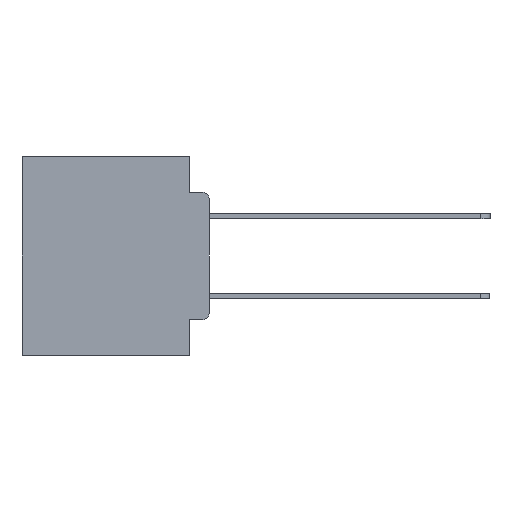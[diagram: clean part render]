
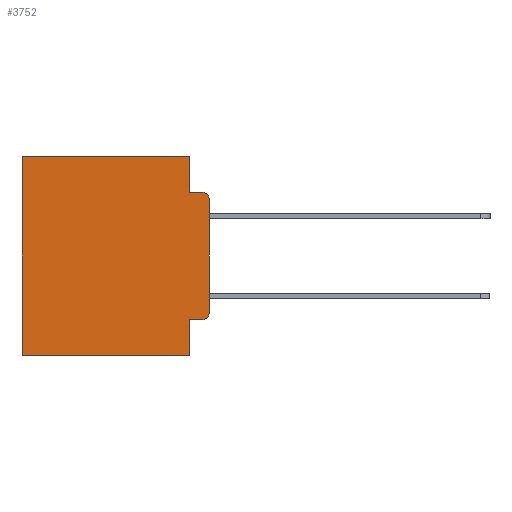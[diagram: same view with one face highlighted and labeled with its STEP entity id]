
A CAD part, left-side view. The second image highlights one B-rep face of the part: STEP entity #3752.
In plain terms, the highlighted planar face has unit normal (-1, 0, 0).
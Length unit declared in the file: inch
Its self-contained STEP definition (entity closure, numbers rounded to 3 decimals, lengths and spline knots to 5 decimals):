
#429 = CARTESIAN_POINT ( 'NONE',  ( 0.298, 0., -0.1085 ) ) ;
#691 = VECTOR ( 'NONE', #7239, 39.37008 ) ;
#1115 = ORIENTED_EDGE ( 'NONE', *, *, #2451, .T. ) ;
#2250 = CARTESIAN_POINT ( 'NONE',  ( 0.298, 0.473, 0. ) ) ;
#2272 = LINE ( 'NONE', #19275, #691 ) ;
#2451 = EDGE_CURVE ( 'NONE', #23999, #26126, #15797, .T. ) ;
#2770 = DIRECTION ( 'NONE',  ( -1., 0., 0. ) ) ;
#2798 = CARTESIAN_POINT ( 'NONE',  ( 0.298, 0., 0. ) ) ;
#3145 = ORIENTED_EDGE ( 'NONE', *, *, #28046, .T. ) ;
#3311 = DIRECTION ( 'NONE',  ( 0., 1., 0. ) ) ;
#3649 = EDGE_LOOP ( 'NONE', ( #17218, #3145, #24891, #10962, #20276, #14297, #28749, #30185, #22831, #1115 ) ) ;
#3752 = ADVANCED_FACE ( 'NONE', ( #28110 ), #26396, .F. ) ;
#4441 = AXIS2_PLACEMENT_3D ( 'NONE', #21143, #28683, #28322 ) ;
#5782 = EDGE_CURVE ( 'NONE', #24346, #23999, #2272, .T. ) ;
#5979 = DIRECTION ( 'NONE',  ( 0., 0., -1. ) ) ;
#6284 = CARTESIAN_POINT ( 'NONE',  ( 0.298, 0.051, -0.0885 ) ) ;
#6443 = DIRECTION ( 'NONE',  ( 0., 0., -1. ) ) ;
#6821 = CARTESIAN_POINT ( 'NONE',  ( 0.298, 0.051, -0.0885 ) ) ;
#7239 = DIRECTION ( 'NONE',  ( 0., -1., 0. ) ) ;
#7537 = LINE ( 'NONE', #23138, #25719 ) ;
#8365 = DIRECTION ( 'NONE',  ( -1., 0., 0. ) ) ;
#8428 = EDGE_CURVE ( 'NONE', #30101, #26126, #12114, .T. ) ;
#8796 = VERTEX_POINT ( 'NONE', #26924 ) ;
#9037 = EDGE_CURVE ( 'NONE', #24346, #30739, #7537, .T. ) ;
#9286 = DIRECTION ( 'NONE',  ( 0., -1., 0. ) ) ;
#10211 = DIRECTION ( 'NONE',  ( 0., 0., -1. ) ) ;
#10731 = EDGE_CURVE ( 'NONE', #30165, #25965, #17637, .T. ) ;
#10962 = ORIENTED_EDGE ( 'NONE', *, *, #18756, .F. ) ;
#11138 = DIRECTION ( 'NONE',  ( 0., 1., 0. ) ) ;
#12114 = LINE ( 'NONE', #2798, #23971 ) ;
#12420 = LINE ( 'NONE', #26131, #24270 ) ;
#13911 = EDGE_CURVE ( 'NONE', #25965, #8796, #14482, .T. ) ;
#14201 = VECTOR ( 'NONE', #9286, 39.37008 ) ;
#14297 = ORIENTED_EDGE ( 'NONE', *, *, #13911, .T. ) ;
#14482 = LINE ( 'NONE', #18027, #27673 ) ;
#14694 = AXIS2_PLACEMENT_3D ( 'NONE', #22663, #8365, #24974 ) ;
#15154 = CARTESIAN_POINT ( 'NONE',  ( 0.298, 0.051, -0.4115 ) ) ;
#15797 = CIRCLE ( 'NONE', #18261, 0.02 ) ;
#17218 = ORIENTED_EDGE ( 'NONE', *, *, #8428, .F. ) ;
#17482 = CARTESIAN_POINT ( 'NONE',  ( 0.298, 0.051, -0.5 ) ) ;
#17637 = LINE ( 'NONE', #27119, #23099 ) ;
#18027 = CARTESIAN_POINT ( 'NONE',  ( 0.298, 0.473, 0. ) ) ;
#18261 = AXIS2_PLACEMENT_3D ( 'NONE', #26994, #2770, #25684 ) ;
#18501 = CARTESIAN_POINT ( 'NONE',  ( 0.298, 0.02, -0.0885 ) ) ;
#18756 = EDGE_CURVE ( 'NONE', #30165, #22189, #12420, .T. ) ;
#19275 = CARTESIAN_POINT ( 'NONE',  ( 0.298, 0.051, -0.4115 ) ) ;
#20276 = ORIENTED_EDGE ( 'NONE', *, *, #10731, .T. ) ;
#20559 = LINE ( 'NONE', #6821, #14201 ) ;
#21086 = VERTEX_POINT ( 'NONE', #18501 ) ;
#21143 = CARTESIAN_POINT ( 'NONE',  ( 0.298, 0., 0. ) ) ;
#22079 = CARTESIAN_POINT ( 'NONE',  ( 0.298, 0., -0.3915 ) ) ;
#22189 = VERTEX_POINT ( 'NONE', #6284 ) ;
#22663 = CARTESIAN_POINT ( 'NONE',  ( 0.298, 0.02, -0.1085 ) ) ;
#22667 = LINE ( 'NONE', #27632, #28078 ) ;
#22831 = ORIENTED_EDGE ( 'NONE', *, *, #5782, .T. ) ;
#23099 = VECTOR ( 'NONE', #3311, 39.37008 ) ;
#23138 = CARTESIAN_POINT ( 'NONE',  ( 0.298, 0.051, 0. ) ) ;
#23394 = EDGE_CURVE ( 'NONE', #22189, #21086, #20559, .T. ) ;
#23935 = CIRCLE ( 'NONE', #14694, 0.02 ) ;
#23971 = VECTOR ( 'NONE', #10211, 39.37008 ) ;
#23999 = VERTEX_POINT ( 'NONE', #30246 ) ;
#24270 = VECTOR ( 'NONE', #28472, 39.37008 ) ;
#24346 = VERTEX_POINT ( 'NONE', #15154 ) ;
#24891 = ORIENTED_EDGE ( 'NONE', *, *, #23394, .F. ) ;
#24974 = DIRECTION ( 'NONE',  ( 0., 0., -1. ) ) ;
#25684 = DIRECTION ( 'NONE',  ( 0., 0., -1. ) ) ;
#25719 = VECTOR ( 'NONE', #6443, 39.37008 ) ;
#25965 = VERTEX_POINT ( 'NONE', #2250 ) ;
#26126 = VERTEX_POINT ( 'NONE', #22079 ) ;
#26131 = CARTESIAN_POINT ( 'NONE',  ( 0.298, 0.051, 0. ) ) ;
#26328 = EDGE_CURVE ( 'NONE', #30739, #8796, #22667, .T. ) ;
#26396 = PLANE ( 'NONE',  #4441 ) ;
#26924 = CARTESIAN_POINT ( 'NONE',  ( 0.298, 0.473, -0.5 ) ) ;
#26979 = CARTESIAN_POINT ( 'NONE',  ( 0.298, 0.051, 0. ) ) ;
#26994 = CARTESIAN_POINT ( 'NONE',  ( 0.298, 0.02, -0.3915 ) ) ;
#27119 = CARTESIAN_POINT ( 'NONE',  ( 0.298, 0., 0. ) ) ;
#27632 = CARTESIAN_POINT ( 'NONE',  ( 0.298, 0., -0.5 ) ) ;
#27673 = VECTOR ( 'NONE', #5979, 39.37008 ) ;
#28046 = EDGE_CURVE ( 'NONE', #30101, #21086, #23935, .T. ) ;
#28078 = VECTOR ( 'NONE', #11138, 39.37008 ) ;
#28110 = FACE_OUTER_BOUND ( 'NONE', #3649, .T. ) ;
#28322 = DIRECTION ( 'NONE',  ( 0., 0., -1. ) ) ;
#28472 = DIRECTION ( 'NONE',  ( 0., 0., -1. ) ) ;
#28683 = DIRECTION ( 'NONE',  ( 1., 0., 0. ) ) ;
#28749 = ORIENTED_EDGE ( 'NONE', *, *, #26328, .F. ) ;
#30101 = VERTEX_POINT ( 'NONE', #429 ) ;
#30165 = VERTEX_POINT ( 'NONE', #26979 ) ;
#30185 = ORIENTED_EDGE ( 'NONE', *, *, #9037, .F. ) ;
#30246 = CARTESIAN_POINT ( 'NONE',  ( 0.298, 0.02, -0.4115 ) ) ;
#30739 = VERTEX_POINT ( 'NONE', #17482 ) ;
